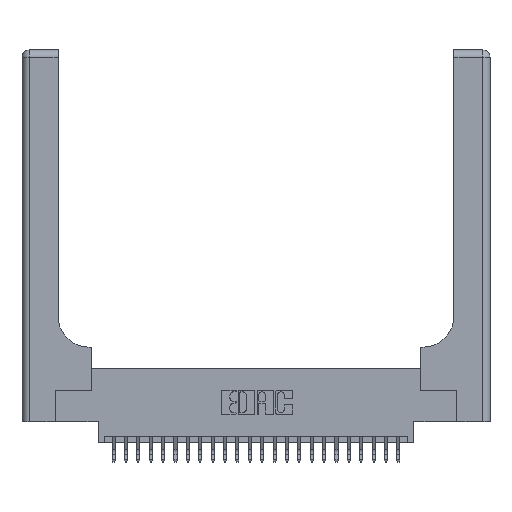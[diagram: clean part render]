
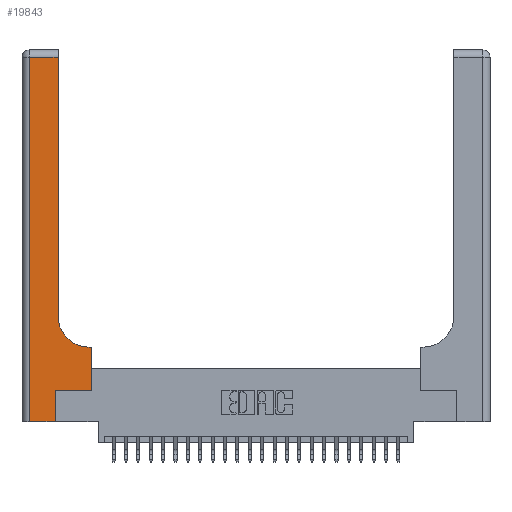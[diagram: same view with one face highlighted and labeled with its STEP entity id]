
A CAD part, top view. The second image highlights one B-rep face of the part: STEP entity #19843.
In plain terms, the highlighted planar face has unit normal (0, 0, 1).
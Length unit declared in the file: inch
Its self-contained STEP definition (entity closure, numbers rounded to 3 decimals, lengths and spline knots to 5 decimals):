
#236 = ORIENTED_EDGE ( 'NONE', *, *, #11423, .T. ) ;
#455 = LINE ( 'NONE', #16217, #6748 ) ;
#821 = EDGE_CURVE ( 'NONE', #2198, #4155, #19778, .T. ) ;
#981 = ORIENTED_EDGE ( 'NONE', *, *, #12071, .T. ) ;
#1151 = VERTEX_POINT ( 'NONE', #4619 ) ;
#1896 = CARTESIAN_POINT ( 'NONE',  ( 0.269, 0.25, 0.37 ) ) ;
#2002 = ORIENTED_EDGE ( 'NONE', *, *, #9097, .T. ) ;
#2198 = VERTEX_POINT ( 'NONE', #24925 ) ;
#4155 = VERTEX_POINT ( 'NONE', #17107 ) ;
#4619 = CARTESIAN_POINT ( 'NONE',  ( 0.2915, 0.85, 0.37 ) ) ;
#4677 = VERTEX_POINT ( 'NONE', #20141 ) ;
#4704 = LINE ( 'NONE', #19424, #26600 ) ;
#4765 = ORIENTED_EDGE ( 'NONE', *, *, #821, .T. ) ;
#4947 = DIRECTION ( 'NONE',  ( 1., 0., 0. ) ) ;
#5271 = AXIS2_PLACEMENT_3D ( 'NONE', #23864, #11741, #25992 ) ;
#6271 = ORIENTED_EDGE ( 'NONE', *, *, #9901, .T. ) ;
#6748 = VECTOR ( 'NONE', #7988, 39.37008 ) ;
#6826 = DIRECTION ( 'NONE',  ( 0., 0., -1. ) ) ;
#6894 = CARTESIAN_POINT ( 'NONE',  ( 0.06, 2.94, 0.37 ) ) ;
#7594 = VECTOR ( 'NONE', #12654, 39.37008 ) ;
#7988 = DIRECTION ( 'NONE',  ( 0., -1., 0. ) ) ;
#8295 = VECTOR ( 'NONE', #15469, 39.37008 ) ;
#9097 = EDGE_CURVE ( 'NONE', #14568, #2198, #24638, .T. ) ;
#9828 = DIRECTION ( 'NONE',  ( 0., 1., 0. ) ) ;
#9901 = EDGE_CURVE ( 'NONE', #12075, #4677, #12175, .T. ) ;
#11423 = EDGE_CURVE ( 'NONE', #4155, #1151, #16893, .T. ) ;
#11518 = VECTOR ( 'NONE', #9828, 39.37008 ) ;
#11741 = DIRECTION ( 'NONE',  ( 0., 0., -1. ) ) ;
#12071 = EDGE_CURVE ( 'NONE', #25019, #12075, #4704, .T. ) ;
#12075 = VERTEX_POINT ( 'NONE', #21464 ) ;
#12175 = LINE ( 'NONE', #26203, #11518 ) ;
#12442 = CARTESIAN_POINT ( 'NONE',  ( 0.2915, 0.6, 0.37 ) ) ;
#12564 = CARTESIAN_POINT ( 'NONE',  ( 0., 2.94, 0.37 ) ) ;
#12654 = DIRECTION ( 'NONE',  ( -1., 0., 0. ) ) ;
#12750 = DIRECTION ( 'NONE',  ( -1., 0., 0. ) ) ;
#13394 = ORIENTED_EDGE ( 'NONE', *, *, #19960, .T. ) ;
#13788 = LINE ( 'NONE', #12564, #7594 ) ;
#14319 = EDGE_CURVE ( 'NONE', #24012, #14515, #13788, .T. ) ;
#14435 = DIRECTION ( 'NONE',  ( 1., 0., 0. ) ) ;
#14515 = VERTEX_POINT ( 'NONE', #6894 ) ;
#14568 = VERTEX_POINT ( 'NONE', #15404 ) ;
#14754 = CARTESIAN_POINT ( 'NONE',  ( 0.06, 0., 0.37 ) ) ;
#14913 = EDGE_CURVE ( 'NONE', #4677, #14568, #15337, .T. ) ;
#15337 = LINE ( 'NONE', #1896, #25517 ) ;
#15404 = CARTESIAN_POINT ( 'NONE',  ( 0.5585, 0.25, 0.37 ) ) ;
#15469 = DIRECTION ( 'NONE',  ( 0., 1., 0. ) ) ;
#15646 = EDGE_LOOP ( 'NONE', ( #17490, #17700, #13394, #981, #6271, #22211, #2002, #4765, #236 ) ) ;
#16217 = CARTESIAN_POINT ( 'NONE',  ( 0.06, 3., 0.37 ) ) ;
#16893 = CIRCLE ( 'NONE', #19679, 0.25 ) ;
#17107 = CARTESIAN_POINT ( 'NONE',  ( 0.5415, 0.6, 0.37 ) ) ;
#17490 = ORIENTED_EDGE ( 'NONE', *, *, #24210, .T. ) ;
#17700 = ORIENTED_EDGE ( 'NONE', *, *, #14319, .T. ) ;
#19186 = CARTESIAN_POINT ( 'NONE',  ( 0.5415, 0.85, 0.37 ) ) ;
#19424 = CARTESIAN_POINT ( 'NONE',  ( 0., 0., 0.37 ) ) ;
#19480 = CARTESIAN_POINT ( 'NONE',  ( 0.5585, 0.25, 0.37 ) ) ;
#19679 = AXIS2_PLACEMENT_3D ( 'NONE', #19186, #6826, #21225 ) ;
#19778 = LINE ( 'NONE', #12442, #25180 ) ;
#19843 = ADVANCED_FACE ( 'NONE', ( #24422 ), #23954, .F. ) ;
#19960 = EDGE_CURVE ( 'NONE', #14515, #25019, #455, .T. ) ;
#20141 = CARTESIAN_POINT ( 'NONE',  ( 0.269, 0.25, 0.37 ) ) ;
#21225 = DIRECTION ( 'NONE',  ( 1., 0., 0. ) ) ;
#21464 = CARTESIAN_POINT ( 'NONE',  ( 0.269, 0., 0.37 ) ) ;
#22211 = ORIENTED_EDGE ( 'NONE', *, *, #14913, .T. ) ;
#23864 = CARTESIAN_POINT ( 'NONE',  ( 0., 3., 0.37 ) ) ;
#23909 = CARTESIAN_POINT ( 'NONE',  ( 0.2915, 2.94, 0.37 ) ) ;
#23954 = PLANE ( 'NONE',  #5271 ) ;
#24012 = VERTEX_POINT ( 'NONE', #23909 ) ;
#24210 = EDGE_CURVE ( 'NONE', #1151, #24012, #26145, .T. ) ;
#24422 = FACE_OUTER_BOUND ( 'NONE', #15646, .T. ) ;
#24509 = CARTESIAN_POINT ( 'NONE',  ( 0.2915, 3., 0.37 ) ) ;
#24638 = LINE ( 'NONE', #19480, #8295 ) ;
#24925 = CARTESIAN_POINT ( 'NONE',  ( 0.5585, 0.6, 0.37 ) ) ;
#25019 = VERTEX_POINT ( 'NONE', #14754 ) ;
#25180 = VECTOR ( 'NONE', #12750, 39.37008 ) ;
#25501 = VECTOR ( 'NONE', #26564, 39.37008 ) ;
#25517 = VECTOR ( 'NONE', #14435, 39.37008 ) ;
#25992 = DIRECTION ( 'NONE',  ( -1., 0., 0. ) ) ;
#26145 = LINE ( 'NONE', #24509, #25501 ) ;
#26203 = CARTESIAN_POINT ( 'NONE',  ( 0.269, 0., 0.37 ) ) ;
#26564 = DIRECTION ( 'NONE',  ( 0., 1., 0. ) ) ;
#26600 = VECTOR ( 'NONE', #4947, 39.37008 ) ;
